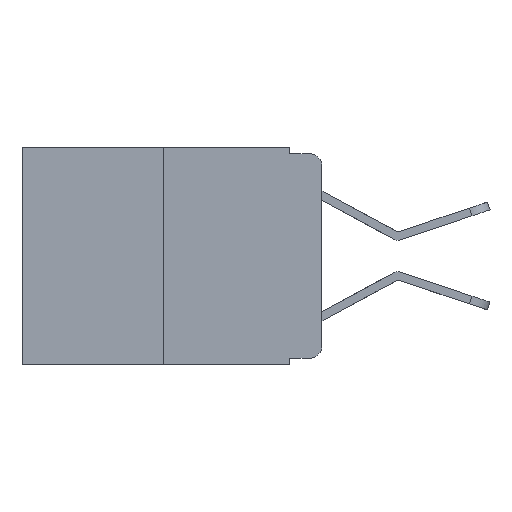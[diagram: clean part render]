
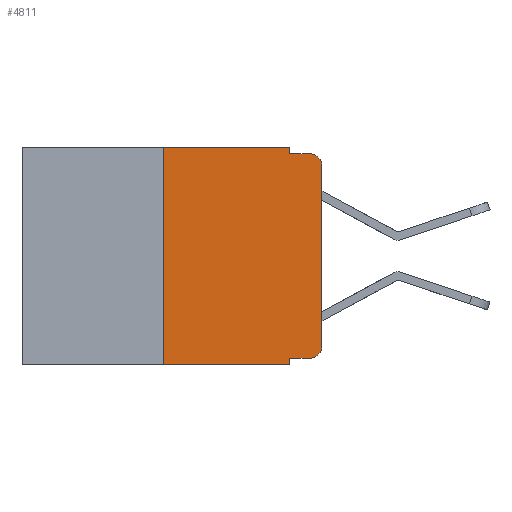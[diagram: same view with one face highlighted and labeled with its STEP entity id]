
A CAD part, left-side view. The second image highlights one B-rep face of the part: STEP entity #4811.
In plain terms, the highlighted planar face has unit normal (-1, 0, 0).
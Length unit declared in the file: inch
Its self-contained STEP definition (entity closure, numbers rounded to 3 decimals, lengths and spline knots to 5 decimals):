
#152 = AXIS2_PLACEMENT_3D ( 'NONE', #3838, #12662, #285 ) ;
#285 = DIRECTION ( 'NONE',  ( 0., 0., -1. ) ) ;
#597 = FACE_OUTER_BOUND ( 'NONE', #4139, .T. ) ;
#623 = VERTEX_POINT ( 'NONE', #7516 ) ;
#706 = CARTESIAN_POINT ( 'NONE',  ( 0., 0.25, 0. ) ) ;
#822 = ORIENTED_EDGE ( 'NONE', *, *, #1695, .T. ) ;
#1111 = ORIENTED_EDGE ( 'NONE', *, *, #10690, .T. ) ;
#1123 = DIRECTION ( 'NONE',  ( -1., 0., 0. ) ) ;
#1232 = VECTOR ( 'NONE', #19389, 39.37008 ) ;
#1452 = CARTESIAN_POINT ( 'NONE',  ( 0., 0.051, -0.01 ) ) ;
#1624 = ORIENTED_EDGE ( 'NONE', *, *, #15304, .F. ) ;
#1695 = EDGE_CURVE ( 'NONE', #4559, #7302, #6906, .T. ) ;
#2011 = LINE ( 'NONE', #18509, #20958 ) ;
#2429 = CARTESIAN_POINT ( 'NONE',  ( 0., 0.051, -0.333 ) ) ;
#2513 = VECTOR ( 'NONE', #14925, 39.37008 ) ;
#2854 = AXIS2_PLACEMENT_3D ( 'NONE', #15832, #15986, #10713 ) ;
#2976 = VERTEX_POINT ( 'NONE', #16351 ) ;
#3130 = CARTESIAN_POINT ( 'NONE',  ( 0., 0.25, -0.343 ) ) ;
#3381 = LINE ( 'NONE', #3492, #15591 ) ;
#3492 = CARTESIAN_POINT ( 'NONE',  ( 0., 0.051, 0. ) ) ;
#3777 = ORIENTED_EDGE ( 'NONE', *, *, #19658, .F. ) ;
#3838 = CARTESIAN_POINT ( 'NONE',  ( 0., 0.473, 0. ) ) ;
#3842 = VERTEX_POINT ( 'NONE', #17061 ) ;
#4056 = DIRECTION ( 'NONE',  ( 0., -1., 0. ) ) ;
#4139 = EDGE_LOOP ( 'NONE', ( #1111, #16374, #1624, #4874, #10592, #3777, #822, #12756, #21207, #4273 ) ) ;
#4184 = EDGE_CURVE ( 'NONE', #21039, #2976, #4308, .T. ) ;
#4273 = ORIENTED_EDGE ( 'NONE', *, *, #5787, .T. ) ;
#4308 = LINE ( 'NONE', #22917, #13431 ) ;
#4559 = VERTEX_POINT ( 'NONE', #3130 ) ;
#4811 = ADVANCED_FACE ( 'NONE', ( #597 ), #10877, .F. ) ;
#4874 = ORIENTED_EDGE ( 'NONE', *, *, #4184, .F. ) ;
#4908 = AXIS2_PLACEMENT_3D ( 'NONE', #4924, #1123, #17387 ) ;
#4924 = CARTESIAN_POINT ( 'NONE',  ( 0., 0.02, -0.03 ) ) ;
#5787 = EDGE_CURVE ( 'NONE', #22279, #3842, #21165, .T. ) ;
#6093 = CARTESIAN_POINT ( 'NONE',  ( 0., 0., -0.03 ) ) ;
#6578 = LINE ( 'NONE', #6985, #1232 ) ;
#6828 = VERTEX_POINT ( 'NONE', #22210 ) ;
#6906 = LINE ( 'NONE', #7777, #19913 ) ;
#6985 = CARTESIAN_POINT ( 'NONE',  ( 0., 0.051, -0.333 ) ) ;
#7302 = VERTEX_POINT ( 'NONE', #7398 ) ;
#7398 = CARTESIAN_POINT ( 'NONE',  ( 0., 0.051, -0.343 ) ) ;
#7516 = CARTESIAN_POINT ( 'NONE',  ( 0., 0.25, 0. ) ) ;
#7722 = EDGE_CURVE ( 'NONE', #18400, #6828, #21882, .T. ) ;
#7777 = CARTESIAN_POINT ( 'NONE',  ( 0., 0.473, -0.343 ) ) ;
#8076 = LINE ( 'NONE', #9357, #16119 ) ;
#8131 = CARTESIAN_POINT ( 'NONE',  ( 0., 0.051, 0. ) ) ;
#8269 = DIRECTION ( 'NONE',  ( 0., 0., 1. ) ) ;
#9029 = EDGE_CURVE ( 'NONE', #10016, #22279, #6578, .T. ) ;
#9357 = CARTESIAN_POINT ( 'NONE',  ( 0., 0.473, 0. ) ) ;
#9430 = DIRECTION ( 'NONE',  ( 0., -1., 0. ) ) ;
#9599 = VECTOR ( 'NONE', #11967, 39.37008 ) ;
#10016 = VERTEX_POINT ( 'NONE', #2429 ) ;
#10309 = LINE ( 'NONE', #706, #2513 ) ;
#10592 = ORIENTED_EDGE ( 'NONE', *, *, #19615, .F. ) ;
#10690 = EDGE_CURVE ( 'NONE', #3842, #18400, #2011, .T. ) ;
#10713 = DIRECTION ( 'NONE',  ( 0., 0., -1. ) ) ;
#10877 = PLANE ( 'NONE',  #152 ) ;
#11967 = DIRECTION ( 'NONE',  ( 0., -1., 0. ) ) ;
#12662 = DIRECTION ( 'NONE',  ( 1., 0., 0. ) ) ;
#12756 = ORIENTED_EDGE ( 'NONE', *, *, #18628, .F. ) ;
#13431 = VECTOR ( 'NONE', #14301, 39.37008 ) ;
#14301 = DIRECTION ( 'NONE',  ( 0., 0., -1. ) ) ;
#14925 = DIRECTION ( 'NONE',  ( 0., 0., 1. ) ) ;
#15304 = EDGE_CURVE ( 'NONE', #2976, #6828, #21533, .T. ) ;
#15356 = CARTESIAN_POINT ( 'NONE',  ( 0., 0.02, -0.333 ) ) ;
#15591 = VECTOR ( 'NONE', #17390, 39.37008 ) ;
#15832 = CARTESIAN_POINT ( 'NONE',  ( 0., 0.02, -0.313 ) ) ;
#15986 = DIRECTION ( 'NONE',  ( -1., 0., 0. ) ) ;
#16119 = VECTOR ( 'NONE', #9430, 39.37008 ) ;
#16351 = CARTESIAN_POINT ( 'NONE',  ( 0., 0.051, -0.01 ) ) ;
#16374 = ORIENTED_EDGE ( 'NONE', *, *, #7722, .T. ) ;
#17061 = CARTESIAN_POINT ( 'NONE',  ( 0., 0., -0.313 ) ) ;
#17387 = DIRECTION ( 'NONE',  ( 0., 0., -1. ) ) ;
#17390 = DIRECTION ( 'NONE',  ( 0., 0., -1. ) ) ;
#18400 = VERTEX_POINT ( 'NONE', #6093 ) ;
#18509 = CARTESIAN_POINT ( 'NONE',  ( 0., 0., 0. ) ) ;
#18628 = EDGE_CURVE ( 'NONE', #10016, #7302, #3381, .T. ) ;
#19389 = DIRECTION ( 'NONE',  ( 0., -1., 0. ) ) ;
#19615 = EDGE_CURVE ( 'NONE', #623, #21039, #8076, .T. ) ;
#19658 = EDGE_CURVE ( 'NONE', #4559, #623, #10309, .T. ) ;
#19913 = VECTOR ( 'NONE', #4056, 39.37008 ) ;
#20958 = VECTOR ( 'NONE', #8269, 39.37008 ) ;
#21039 = VERTEX_POINT ( 'NONE', #8131 ) ;
#21165 = CIRCLE ( 'NONE', #2854, 0.02 ) ;
#21207 = ORIENTED_EDGE ( 'NONE', *, *, #9029, .T. ) ;
#21533 = LINE ( 'NONE', #1452, #9599 ) ;
#21882 = CIRCLE ( 'NONE', #4908, 0.02 ) ;
#22210 = CARTESIAN_POINT ( 'NONE',  ( 0., 0.02, -0.01 ) ) ;
#22279 = VERTEX_POINT ( 'NONE', #15356 ) ;
#22917 = CARTESIAN_POINT ( 'NONE',  ( 0., 0.051, 0. ) ) ;
